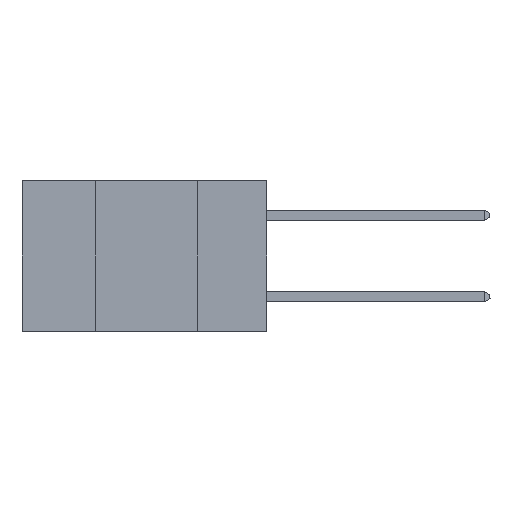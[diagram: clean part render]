
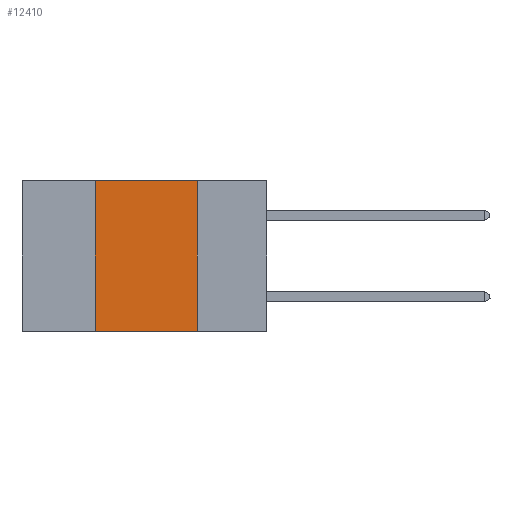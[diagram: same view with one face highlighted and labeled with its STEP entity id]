
A CAD part, left-side view. The second image highlights one B-rep face of the part: STEP entity #12410.
In plain terms, the highlighted planar face has unit normal (-1, 0, 0).
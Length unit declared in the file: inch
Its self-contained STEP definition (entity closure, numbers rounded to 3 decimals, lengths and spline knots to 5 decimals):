
#6 = EDGE_CURVE ( 'NONE', #3172, #21704, #13320, .T. ) ;
#1782 = CARTESIAN_POINT ( 'NONE',  ( 0., 0.17, 0. ) ) ;
#2228 = DIRECTION ( 'NONE',  ( 1., 0., 0. ) ) ;
#2252 = CARTESIAN_POINT ( 'NONE',  ( 0., 0.6, -0.37 ) ) ;
#2459 = VERTEX_POINT ( 'NONE', #7670 ) ;
#3172 = VERTEX_POINT ( 'NONE', #18351 ) ;
#3456 = DIRECTION ( 'NONE',  ( 0., 0., -1. ) ) ;
#3910 = CARTESIAN_POINT ( 'NONE',  ( 0., 0.6, 0. ) ) ;
#4732 = LINE ( 'NONE', #1782, #6602 ) ;
#5091 = CARTESIAN_POINT ( 'NONE',  ( 0., 0.6, 0. ) ) ;
#5184 = VERTEX_POINT ( 'NONE', #11707 ) ;
#5554 = EDGE_CURVE ( 'NONE', #5184, #2459, #16068, .T. ) ;
#5939 = ORIENTED_EDGE ( 'NONE', *, *, #6, .T. ) ;
#6056 = EDGE_CURVE ( 'NONE', #2459, #21704, #4732, .T. ) ;
#6602 = VECTOR ( 'NONE', #3456, 39.37008 ) ;
#7670 = CARTESIAN_POINT ( 'NONE',  ( 0., 0.17, 0. ) ) ;
#8323 = DIRECTION ( 'NONE',  ( 0., -1., 0. ) ) ;
#8917 = DIRECTION ( 'NONE',  ( 0., 0., -1. ) ) ;
#9330 = ORIENTED_EDGE ( 'NONE', *, *, #19625, .F. ) ;
#10115 = AXIS2_PLACEMENT_3D ( 'NONE', #3910, #2228, #8917 ) ;
#10768 = PLANE ( 'NONE',  #10115 ) ;
#10788 = DIRECTION ( 'NONE',  ( 0., -1., 0. ) ) ;
#11707 = CARTESIAN_POINT ( 'NONE',  ( 0., 0.42, 0. ) ) ;
#12410 = ADVANCED_FACE ( 'NONE', ( #16890 ), #10768, .F. ) ;
#12873 = CARTESIAN_POINT ( 'NONE',  ( 0., 0.17, -0.37 ) ) ;
#13320 = LINE ( 'NONE', #2252, #20591 ) ;
#13693 = EDGE_LOOP ( 'NONE', ( #18156, #20642, #9330, #5939 ) ) ;
#15028 = VECTOR ( 'NONE', #15318, 39.37008 ) ;
#15161 = CARTESIAN_POINT ( 'NONE',  ( 0., 0.42, 0. ) ) ;
#15318 = DIRECTION ( 'NONE',  ( 0., 0., 1. ) ) ;
#16068 = LINE ( 'NONE', #5091, #19091 ) ;
#16870 = LINE ( 'NONE', #15161, #15028 ) ;
#16890 = FACE_OUTER_BOUND ( 'NONE', #13693, .T. ) ;
#18156 = ORIENTED_EDGE ( 'NONE', *, *, #6056, .F. ) ;
#18351 = CARTESIAN_POINT ( 'NONE',  ( 0., 0.42, -0.37 ) ) ;
#19091 = VECTOR ( 'NONE', #8323, 39.37008 ) ;
#19625 = EDGE_CURVE ( 'NONE', #3172, #5184, #16870, .T. ) ;
#20591 = VECTOR ( 'NONE', #10788, 39.37008 ) ;
#20642 = ORIENTED_EDGE ( 'NONE', *, *, #5554, .F. ) ;
#21704 = VERTEX_POINT ( 'NONE', #12873 ) ;
